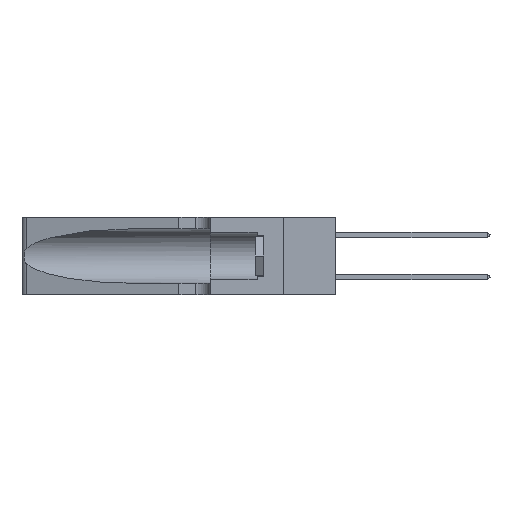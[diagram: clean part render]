
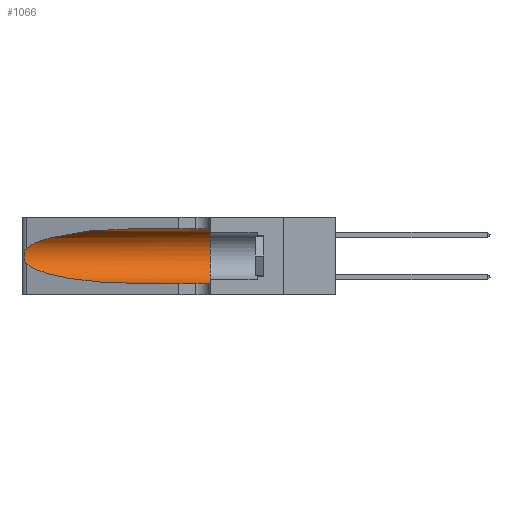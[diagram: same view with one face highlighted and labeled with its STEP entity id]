
A CAD part, left-side view. The second image highlights one B-rep face of the part: STEP entity #1066.
In plain terms, the highlighted cylindrical face has radius 3.308 mm (diameter 6.617 mm), a partial arc.
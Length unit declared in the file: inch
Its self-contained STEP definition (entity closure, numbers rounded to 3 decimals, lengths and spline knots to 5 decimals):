
#169 = B_SPLINE_CURVE_WITH_KNOTS ( 'NONE', 3,
 ( #1000, #22191, #11806, #26353, #13936, #1096, #16055, #3280, #18119, #5422, #20184, #7580, #22273, #9758 ),
 .UNSPECIFIED., .F., .F.,
 ( 4, 2, 2, 2, 2, 2, 4 ),
 ( 0., 0.00027, 0.00053, 0.00107, 0.0016, 0.00187, 0.00214 ),
 .UNSPECIFIED. ) ;
#186 = AXIS2_PLACEMENT_3D ( 'NONE', #985, #15961, #3174 ) ;
#224 = VERTEX_POINT ( 'NONE', #22306 ) ;
#831 = ORIENTED_EDGE ( 'NONE', *, *, #5004, .T. ) ;
#893 = EDGE_CURVE ( 'NONE', #2561, #11177, #25559, .T. ) ;
#909 = CARTESIAN_POINT ( 'NONE',  ( 0.25487, 1.22718, 0.22369 ) ) ;
#985 = CARTESIAN_POINT ( 'NONE',  ( 0.1305, 0.35, 0.185 ) ) ;
#1000 = CARTESIAN_POINT ( 'NONE',  ( 0.25487, 1.22718, 0.22369 ) ) ;
#1066 = ADVANCED_FACE ( 'NONE', ( #16930 ), #16257, .F. ) ;
#1096 = CARTESIAN_POINT ( 'NONE',  ( 0.26018, 1.23835, 0.19895 ) ) ;
#1325 = CARTESIAN_POINT ( 'NONE',  ( 0.1305, 0.35, 0.31525 ) ) ;
#1352 = ORIENTED_EDGE ( 'NONE', *, *, #6690, .F. ) ;
#2561 = VERTEX_POINT ( 'NONE', #20484 ) ;
#3174 = DIRECTION ( 'NONE',  ( 0., 0., 1. ) ) ;
#3280 = CARTESIAN_POINT ( 'NONE',  ( 0.26075, 1.23896, 0.178 ) ) ;
#3868 = DIRECTION ( 'NONE',  ( 0., -1., 0. ) ) ;
#4110 = DIRECTION ( 'NONE',  ( 0., -1., 0. ) ) ;
#4216 = CARTESIAN_POINT ( 'NONE',  ( 0.1305, 1.61858, 0.185 ) ) ;
#4313 = DIRECTION ( 'NONE',  ( 0., 0., -1. ) ) ;
#5004 = EDGE_CURVE ( 'NONE', #11177, #9224, #11425, .T. ) ;
#5422 = CARTESIAN_POINT ( 'NONE',  ( 0.25856, 1.23593, 0.16098 ) ) ;
#6539 = ORIENTED_EDGE ( 'NONE', *, *, #15898, .T. ) ;
#6690 = EDGE_CURVE ( 'NONE', #17209, #9224, #15749, .T. ) ;
#6751 = VERTEX_POINT ( 'NONE', #7662 ) ;
#7481 = EDGE_CURVE ( 'NONE', #6751, #17209, #19567, .T. ) ;
#7580 = CARTESIAN_POINT ( 'NONE',  ( 0.25639, 1.23186, 0.15144 ) ) ;
#7662 = CARTESIAN_POINT ( 'NONE',  ( 0.1305, 0.72297, 0.31525 ) ) ;
#9224 = VERTEX_POINT ( 'NONE', #13825 ) ;
#9758 = CARTESIAN_POINT ( 'NONE',  ( 0.25487, 1.22718, 0.14631 ) ) ;
#9851 = ORIENTED_EDGE ( 'NONE', *, *, #11188, .T. ) ;
#10150 = CARTESIAN_POINT ( 'NONE',  ( 0.1305, 0.72297, 0.05475 ) ) ;
#10182 =( BOUNDED_CURVE ( )  B_SPLINE_CURVE ( 3, ( #24082, #26168, #13761, #909 ),
 .UNSPECIFIED., .F., .F. ) 
 B_SPLINE_CURVE_WITH_KNOTS ( ( 4, 4 ),
 ( 1.5708, 2.84003 ),
 .UNSPECIFIED. ) 
 CURVE ( )  GEOMETRIC_REPRESENTATION_ITEM ( )  RATIONAL_B_SPLINE_CURVE ( ( 1., 0.87, 0.87, 1. ) ) 
 REPRESENTATION_ITEM ( '' )  );
#10241 = CARTESIAN_POINT ( 'NONE',  ( 0.25487, 1.22718, 0.14631 ) ) ;
#10319 = CARTESIAN_POINT ( 'NONE',  ( 0.2373, 1.15595, 0.08982 ) ) ;
#10383 = CARTESIAN_POINT ( 'NONE',  ( 0.18966, 0.96281, 0.05475 ) ) ;
#11177 = VERTEX_POINT ( 'NONE', #20096 ) ;
#11188 = EDGE_CURVE ( 'NONE', #224, #2561, #169, .T. ) ;
#11246 = ORIENTED_EDGE ( 'NONE', *, *, #893, .T. ) ;
#11425 = LINE ( 'NONE', #12637, #21858 ) ;
#11806 = CARTESIAN_POINT ( 'NONE',  ( 0.25639, 1.23184, 0.21858 ) ) ;
#12627 = DIRECTION ( 'NONE',  ( 0., -1., 0. ) ) ;
#12637 = CARTESIAN_POINT ( 'NONE',  ( 0.1305, 1.61858, 0.05475 ) ) ;
#12686 = EDGE_LOOP ( 'NONE', ( #6539, #9851, #11246, #831, #1352, #25916 ) ) ;
#13761 = CARTESIAN_POINT ( 'NONE',  ( 0.2373, 1.15595, 0.28018 ) ) ;
#13825 = CARTESIAN_POINT ( 'NONE',  ( 0.1305, 0.35, 0.05475 ) ) ;
#13936 = CARTESIAN_POINT ( 'NONE',  ( 0.25854, 1.2359, 0.20912 ) ) ;
#14735 = VECTOR ( 'NONE', #12627, 39.37008 ) ;
#15749 = CIRCLE ( 'NONE', #186, 0.13025 ) ;
#15898 = EDGE_CURVE ( 'NONE', #6751, #224, #10182, .T. ) ;
#15961 = DIRECTION ( 'NONE',  ( 0., 1., 0. ) ) ;
#16045 = AXIS2_PLACEMENT_3D ( 'NONE', #4216, #3868, #4313 ) ;
#16055 = CARTESIAN_POINT ( 'NONE',  ( 0.26075, 1.23896, 0.19203 ) ) ;
#16257 = CYLINDRICAL_SURFACE ( 'NONE', #16045, 0.13025 ) ;
#16930 = FACE_OUTER_BOUND ( 'NONE', #12686, .T. ) ;
#17209 = VERTEX_POINT ( 'NONE', #1325 ) ;
#18119 = CARTESIAN_POINT ( 'NONE',  ( 0.26017, 1.23833, 0.17102 ) ) ;
#19567 = LINE ( 'NONE', #25049, #14735 ) ;
#20096 = CARTESIAN_POINT ( 'NONE',  ( 0.1305, 0.72297, 0.05475 ) ) ;
#20184 = CARTESIAN_POINT ( 'NONE',  ( 0.25789, 1.23486, 0.15765 ) ) ;
#20484 = CARTESIAN_POINT ( 'NONE',  ( 0.25487, 1.22718, 0.14631 ) ) ;
#21858 = VECTOR ( 'NONE', #4110, 39.37008 ) ;
#22191 = CARTESIAN_POINT ( 'NONE',  ( 0.25555, 1.22994, 0.2215 ) ) ;
#22273 = CARTESIAN_POINT ( 'NONE',  ( 0.25555, 1.22993, 0.14849 ) ) ;
#22306 = CARTESIAN_POINT ( 'NONE',  ( 0.25487, 1.22718, 0.22369 ) ) ;
#24082 = CARTESIAN_POINT ( 'NONE',  ( 0.1305, 0.72297, 0.31525 ) ) ;
#25049 = CARTESIAN_POINT ( 'NONE',  ( 0.1305, 1.61858, 0.31525 ) ) ;
#25559 =( BOUNDED_CURVE ( )  B_SPLINE_CURVE ( 3, ( #10241, #10319, #10383, #10150 ),
 .UNSPECIFIED., .F., .F. ) 
 B_SPLINE_CURVE_WITH_KNOTS ( ( 4, 4 ),
 ( 3.44316, 4.71239 ),
 .UNSPECIFIED. ) 
 CURVE ( )  GEOMETRIC_REPRESENTATION_ITEM ( )  RATIONAL_B_SPLINE_CURVE ( ( 1., 0.87, 0.87, 1. ) ) 
 REPRESENTATION_ITEM ( '' )  );
#25916 = ORIENTED_EDGE ( 'NONE', *, *, #7481, .F. ) ;
#26168 = CARTESIAN_POINT ( 'NONE',  ( 0.18966, 0.96281, 0.31525 ) ) ;
#26353 = CARTESIAN_POINT ( 'NONE',  ( 0.25787, 1.23484, 0.2124 ) ) ;
